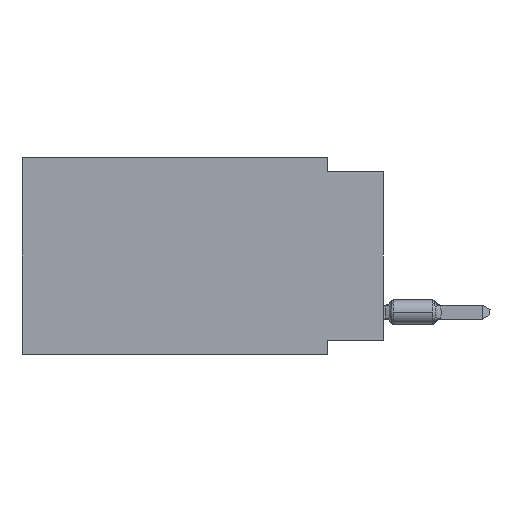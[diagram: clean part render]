
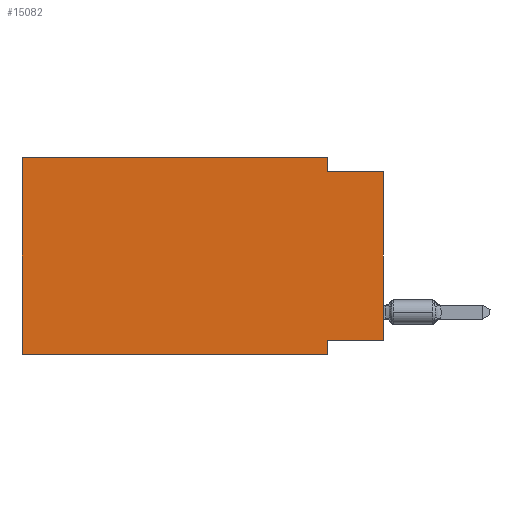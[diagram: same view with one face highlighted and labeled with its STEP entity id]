
A CAD part, left-side view. The second image highlights one B-rep face of the part: STEP entity #15082.
In plain terms, the highlighted planar face has unit normal (-1, 0, 0).
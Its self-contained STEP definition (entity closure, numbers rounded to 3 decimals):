
#177 = CARTESIAN_POINT ( 'NONE',  ( 0., 0., -8.255 ) ) ;
#1409 = LINE ( 'NONE', #3073, #8367 ) ;
#1512 = DIRECTION ( 'NONE',  ( 0., 0., -1. ) ) ;
#1643 = CARTESIAN_POINT ( 'NONE',  ( 0., 2.54, -8.89 ) ) ;
#1889 = EDGE_CURVE ( 'NONE', #20684, #1999, #20984, .T. ) ;
#1965 = CARTESIAN_POINT ( 'NONE',  ( 0., 2.54, -0.635 ) ) ;
#1999 = VERTEX_POINT ( 'NONE', #16926 ) ;
#2758 = DIRECTION ( 'NONE',  ( 0., 0., 1. ) ) ;
#3073 = CARTESIAN_POINT ( 'NONE',  ( 0., 0., -0.635 ) ) ;
#3200 = DIRECTION ( 'NONE',  ( 0., -1., 0. ) ) ;
#4397 = DIRECTION ( 'NONE',  ( 1., 0., 0. ) ) ;
#4646 = VERTEX_POINT ( 'NONE', #13634 ) ;
#4671 = FACE_OUTER_BOUND ( 'NONE', #19950, .T. ) ;
#4923 = ORIENTED_EDGE ( 'NONE', *, *, #15458, .T. ) ;
#6212 = LINE ( 'NONE', #1643, #24873 ) ;
#6258 = ORIENTED_EDGE ( 'NONE', *, *, #27223, .F. ) ;
#6331 = VERTEX_POINT ( 'NONE', #18054 ) ;
#6348 = PLANE ( 'NONE',  #19144 ) ;
#8027 = LINE ( 'NONE', #26325, #24208 ) ;
#8367 = VECTOR ( 'NONE', #3200, 1000. ) ;
#8714 = CARTESIAN_POINT ( 'NONE',  ( 0., 16.383, 0. ) ) ;
#8729 = ORIENTED_EDGE ( 'NONE', *, *, #1889, .F. ) ;
#8788 = DIRECTION ( 'NONE',  ( 0., 1., 0. ) ) ;
#9306 = EDGE_CURVE ( 'NONE', #11235, #19954, #1409, .T. ) ;
#11235 = VERTEX_POINT ( 'NONE', #1965 ) ;
#11633 = VECTOR ( 'NONE', #2758, 1000. ) ;
#12307 = LINE ( 'NONE', #18662, #21562 ) ;
#12382 = CARTESIAN_POINT ( 'NONE',  ( 0., 2.54, 0. ) ) ;
#12452 = DIRECTION ( 'NONE',  ( 0., -1., 0. ) ) ;
#12724 = CARTESIAN_POINT ( 'NONE',  ( 0., 16.383, -8.89 ) ) ;
#12728 = DIRECTION ( 'NONE',  ( 0., 0., -1. ) ) ;
#12874 = VERTEX_POINT ( 'NONE', #18907 ) ;
#13414 = VECTOR ( 'NONE', #14456, 1000. ) ;
#13634 = CARTESIAN_POINT ( 'NONE',  ( 0., 16.383, 0. ) ) ;
#14456 = DIRECTION ( 'NONE',  ( 0., 0., -1. ) ) ;
#14612 = ORIENTED_EDGE ( 'NONE', *, *, #27296, .F. ) ;
#14893 = EDGE_CURVE ( 'NONE', #1999, #6331, #6212, .T. ) ;
#15082 = ADVANCED_FACE ( 'NONE', ( #4671 ), #6348, .F. ) ;
#15458 = EDGE_CURVE ( 'NONE', #20684, #19954, #24225, .T. ) ;
#15598 = VECTOR ( 'NONE', #8788, 1000. ) ;
#15686 = ORIENTED_EDGE ( 'NONE', *, *, #27144, .T. ) ;
#16521 = LINE ( 'NONE', #12382, #13414 ) ;
#16926 = CARTESIAN_POINT ( 'NONE',  ( 0., 2.54, -8.255 ) ) ;
#17322 = EDGE_CURVE ( 'NONE', #12874, #11235, #16521, .T. ) ;
#17328 = CARTESIAN_POINT ( 'NONE',  ( 0., 16.383, -8.89 ) ) ;
#18054 = CARTESIAN_POINT ( 'NONE',  ( 0., 2.54, -8.89 ) ) ;
#18456 = VECTOR ( 'NONE', #21633, 1000. ) ;
#18662 = CARTESIAN_POINT ( 'NONE',  ( 0., 16.383, 0. ) ) ;
#18907 = CARTESIAN_POINT ( 'NONE',  ( 0., 2.54, 0. ) ) ;
#19144 = AXIS2_PLACEMENT_3D ( 'NONE', #8714, #4397, #12728 ) ;
#19620 = CARTESIAN_POINT ( 'NONE',  ( 0., 0., -0.635 ) ) ;
#19950 = EDGE_LOOP ( 'NONE', ( #4923, #23374, #25267, #14612, #6258, #15686, #26488, #8729 ) ) ;
#19954 = VERTEX_POINT ( 'NONE', #19620 ) ;
#20684 = VERTEX_POINT ( 'NONE', #23521 ) ;
#20984 = LINE ( 'NONE', #177, #15598 ) ;
#21562 = VECTOR ( 'NONE', #24631, 1000. ) ;
#21633 = DIRECTION ( 'NONE',  ( 0., -1., 0. ) ) ;
#23374 = ORIENTED_EDGE ( 'NONE', *, *, #9306, .F. ) ;
#23521 = CARTESIAN_POINT ( 'NONE',  ( 0., 0., -8.255 ) ) ;
#23978 = LINE ( 'NONE', #17328, #18456 ) ;
#24178 = VERTEX_POINT ( 'NONE', #12724 ) ;
#24208 = VECTOR ( 'NONE', #12452, 1000. ) ;
#24225 = LINE ( 'NONE', #26432, #11633 ) ;
#24631 = DIRECTION ( 'NONE',  ( 0., 0., 1. ) ) ;
#24873 = VECTOR ( 'NONE', #1512, 1000. ) ;
#25267 = ORIENTED_EDGE ( 'NONE', *, *, #17322, .F. ) ;
#26325 = CARTESIAN_POINT ( 'NONE',  ( 0., 16.383, 0. ) ) ;
#26432 = CARTESIAN_POINT ( 'NONE',  ( 0., 0., 0. ) ) ;
#26488 = ORIENTED_EDGE ( 'NONE', *, *, #14893, .F. ) ;
#27144 = EDGE_CURVE ( 'NONE', #24178, #6331, #23978, .T. ) ;
#27223 = EDGE_CURVE ( 'NONE', #24178, #4646, #12307, .T. ) ;
#27296 = EDGE_CURVE ( 'NONE', #4646, #12874, #8027, .T. ) ;
